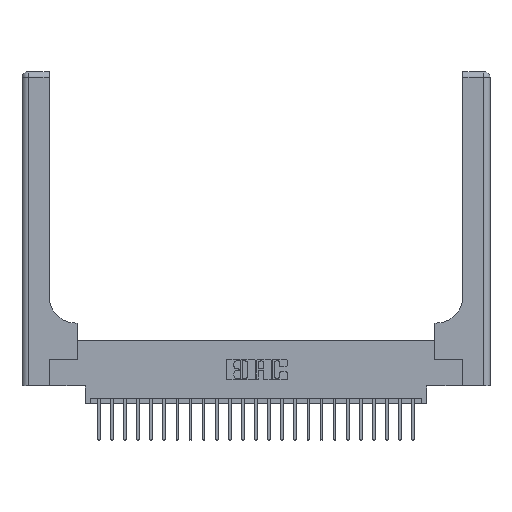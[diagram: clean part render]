
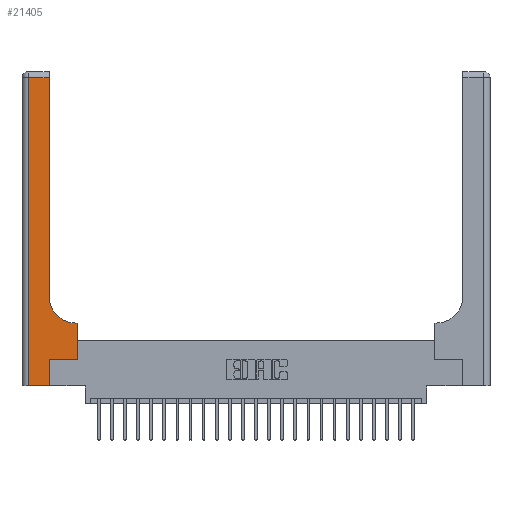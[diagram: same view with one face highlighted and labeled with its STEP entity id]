
A CAD part, top view. The second image highlights one B-rep face of the part: STEP entity #21405.
In plain terms, the highlighted planar face has unit normal (0, 0, 1).
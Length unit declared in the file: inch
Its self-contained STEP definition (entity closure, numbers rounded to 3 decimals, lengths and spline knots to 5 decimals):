
#24 = DIRECTION ( 'NONE',  ( 1., 0., 0. ) ) ;
#36 = DIRECTION ( 'NONE',  ( -1., 0., 0. ) ) ;
#63 = CARTESIAN_POINT ( 'NONE',  ( 0., 0., 0.37 ) ) ;
#169 = VECTOR ( 'NONE', #22784, 39.37008 ) ;
#781 = DIRECTION ( 'NONE',  ( 0., 1., 0. ) ) ;
#1206 = CARTESIAN_POINT ( 'NONE',  ( 0.265, 0.25, 0.37 ) ) ;
#1402 = CARTESIAN_POINT ( 'NONE',  ( 0.528, 0.25, 0.37 ) ) ;
#1836 = ORIENTED_EDGE ( 'NONE', *, *, #12973, .T. ) ;
#1901 = VERTEX_POINT ( 'NONE', #3996 ) ;
#2251 = VECTOR ( 'NONE', #16168, 39.37008 ) ;
#3351 = AXIS2_PLACEMENT_3D ( 'NONE', #3438, #16461, #5329 ) ;
#3438 = CARTESIAN_POINT ( 'NONE',  ( 0.51, 0.85, 0.37 ) ) ;
#3572 = VERTEX_POINT ( 'NONE', #5178 ) ;
#3882 = ORIENTED_EDGE ( 'NONE', *, *, #7866, .T. ) ;
#3996 = CARTESIAN_POINT ( 'NONE',  ( 0.265, 0., 0.37 ) ) ;
#4039 = ORIENTED_EDGE ( 'NONE', *, *, #15456, .T. ) ;
#4217 = LINE ( 'NONE', #63, #18465 ) ;
#4259 = LINE ( 'NONE', #9377, #15940 ) ;
#4453 = CARTESIAN_POINT ( 'NONE',  ( 0.06, 0., 0.37 ) ) ;
#4638 = ORIENTED_EDGE ( 'NONE', *, *, #19518, .T. ) ;
#5178 = CARTESIAN_POINT ( 'NONE',  ( 0.51, 0.6, 0.37 ) ) ;
#5211 = LINE ( 'NONE', #22957, #19463 ) ;
#5329 = DIRECTION ( 'NONE',  ( 1., 0., 0. ) ) ;
#5538 = LINE ( 'NONE', #10937, #19769 ) ;
#6296 = AXIS2_PLACEMENT_3D ( 'NONE', #16203, #21684, #10678 ) ;
#6361 = VERTEX_POINT ( 'NONE', #1206 ) ;
#6495 = LINE ( 'NONE', #7483, #7092 ) ;
#7092 = VECTOR ( 'NONE', #23935, 39.37008 ) ;
#7483 = CARTESIAN_POINT ( 'NONE',  ( 0.06, 3., 0.37 ) ) ;
#7644 = VERTEX_POINT ( 'NONE', #12279 ) ;
#7768 = VERTEX_POINT ( 'NONE', #14620 ) ;
#7866 = EDGE_CURVE ( 'NONE', #9337, #1901, #4217, .T. ) ;
#9337 = VERTEX_POINT ( 'NONE', #4453 ) ;
#9377 = CARTESIAN_POINT ( 'NONE',  ( 0.265, 0.25, 0.37 ) ) ;
#9563 = EDGE_CURVE ( 'NONE', #10607, #17914, #17091, .T. ) ;
#10006 = CARTESIAN_POINT ( 'NONE',  ( 0.26, 2.94, 0.37 ) ) ;
#10607 = VERTEX_POINT ( 'NONE', #1402 ) ;
#10629 = ORIENTED_EDGE ( 'NONE', *, *, #14229, .T. ) ;
#10670 = FACE_OUTER_BOUND ( 'NONE', #17240, .T. ) ;
#10678 = DIRECTION ( 'NONE',  ( -1., 0., 0. ) ) ;
#10937 = CARTESIAN_POINT ( 'NONE',  ( 0., 2.94, 0.37 ) ) ;
#11286 = DIRECTION ( 'NONE',  ( 1., 0., 0. ) ) ;
#11447 = EDGE_CURVE ( 'NONE', #6361, #10607, #4259, .T. ) ;
#11653 = CARTESIAN_POINT ( 'NONE',  ( 0.26, 3., 0.37 ) ) ;
#12279 = CARTESIAN_POINT ( 'NONE',  ( 0.06, 2.94, 0.37 ) ) ;
#12973 = EDGE_CURVE ( 'NONE', #3572, #7768, #16144, .T. ) ;
#13116 = CARTESIAN_POINT ( 'NONE',  ( 0.26, 0.6, 0.37 ) ) ;
#14229 = EDGE_CURVE ( 'NONE', #7644, #9337, #6495, .T. ) ;
#14620 = CARTESIAN_POINT ( 'NONE',  ( 0.26, 0.85, 0.37 ) ) ;
#15065 = LINE ( 'NONE', #11653, #169 ) ;
#15456 = EDGE_CURVE ( 'NONE', #20620, #7644, #5538, .T. ) ;
#15940 = VECTOR ( 'NONE', #24, 39.37008 ) ;
#16144 = CIRCLE ( 'NONE', #3351, 0.25 ) ;
#16168 = DIRECTION ( 'NONE',  ( 0., 1., 0. ) ) ;
#16203 = CARTESIAN_POINT ( 'NONE',  ( 0., 3., 0.37 ) ) ;
#16461 = DIRECTION ( 'NONE',  ( 0., 0., -1. ) ) ;
#17091 = LINE ( 'NONE', #23453, #2251 ) ;
#17240 = EDGE_LOOP ( 'NONE', ( #18719, #4039, #10629, #3882, #4638, #23094, #17846, #18851, #1836 ) ) ;
#17846 = ORIENTED_EDGE ( 'NONE', *, *, #9563, .T. ) ;
#17914 = VERTEX_POINT ( 'NONE', #19397 ) ;
#18207 = VECTOR ( 'NONE', #36, 39.37008 ) ;
#18465 = VECTOR ( 'NONE', #11286, 39.37008 ) ;
#18719 = ORIENTED_EDGE ( 'NONE', *, *, #19953, .T. ) ;
#18851 = ORIENTED_EDGE ( 'NONE', *, *, #20999, .T. ) ;
#19397 = CARTESIAN_POINT ( 'NONE',  ( 0.528, 0.6, 0.37 ) ) ;
#19463 = VECTOR ( 'NONE', #781, 39.37008 ) ;
#19518 = EDGE_CURVE ( 'NONE', #1901, #6361, #5211, .T. ) ;
#19769 = VECTOR ( 'NONE', #23876, 39.37008 ) ;
#19953 = EDGE_CURVE ( 'NONE', #7768, #20620, #15065, .T. ) ;
#20620 = VERTEX_POINT ( 'NONE', #10006 ) ;
#20999 = EDGE_CURVE ( 'NONE', #17914, #3572, #23028, .T. ) ;
#21405 = ADVANCED_FACE ( 'NONE', ( #10670 ), #21607, .F. ) ;
#21607 = PLANE ( 'NONE',  #6296 ) ;
#21684 = DIRECTION ( 'NONE',  ( 0., 0., -1. ) ) ;
#22784 = DIRECTION ( 'NONE',  ( 0., 1., 0. ) ) ;
#22957 = CARTESIAN_POINT ( 'NONE',  ( 0.265, 0., 0.37 ) ) ;
#23028 = LINE ( 'NONE', #13116, #18207 ) ;
#23094 = ORIENTED_EDGE ( 'NONE', *, *, #11447, .T. ) ;
#23453 = CARTESIAN_POINT ( 'NONE',  ( 0.528, 0.25, 0.37 ) ) ;
#23876 = DIRECTION ( 'NONE',  ( -1., 0., 0. ) ) ;
#23935 = DIRECTION ( 'NONE',  ( 0., -1., 0. ) ) ;
